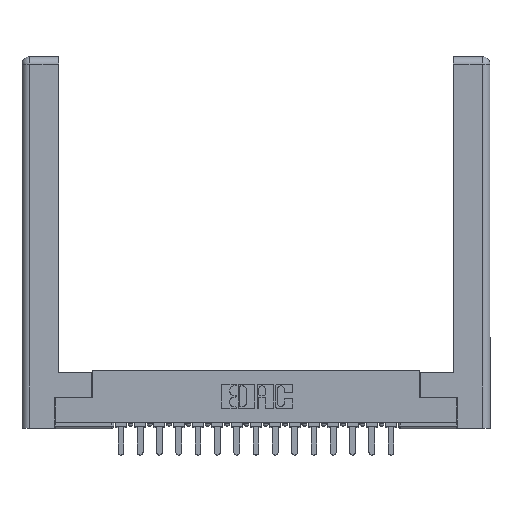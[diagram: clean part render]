
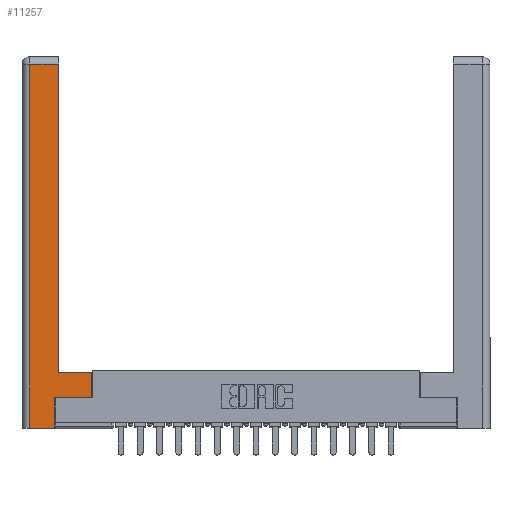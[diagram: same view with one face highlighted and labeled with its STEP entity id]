
A CAD part, top view. The second image highlights one B-rep face of the part: STEP entity #11257.
In plain terms, the highlighted planar face has unit normal (0, 0, 1).
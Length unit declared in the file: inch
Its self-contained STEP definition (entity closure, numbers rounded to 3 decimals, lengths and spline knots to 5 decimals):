
#6 = LINE ( 'NONE', #11619, #14843 ) ;
#325 = LINE ( 'NONE', #17585, #9475 ) ;
#982 = ORIENTED_EDGE ( 'NONE', *, *, #18937, .T. ) ;
#1104 = LINE ( 'NONE', #11465, #16669 ) ;
#1162 = LINE ( 'NONE', #10552, #17207 ) ;
#1489 = EDGE_LOOP ( 'NONE', ( #7624, #16201, #18060, #9174, #8798, #18848, #982, #4136 ) ) ;
#1714 = CARTESIAN_POINT ( 'NONE',  ( 0.295, 0.45, 0. ) ) ;
#1794 = EDGE_CURVE ( 'NONE', #12138, #5463, #15295, .T. ) ;
#2558 = CARTESIAN_POINT ( 'NONE',  ( 0.565, 0.45, 0. ) ) ;
#2696 = EDGE_CURVE ( 'NONE', #5463, #11904, #1104, .T. ) ;
#2821 = VERTEX_POINT ( 'NONE', #5671 ) ;
#2945 = CARTESIAN_POINT ( 'NONE',  ( 0.565, 0.45, 0. ) ) ;
#3159 = CARTESIAN_POINT ( 'NONE',  ( 0.565, 0.245, 0. ) ) ;
#3393 = DIRECTION ( 'NONE',  ( 0., -1., 0. ) ) ;
#3625 = EDGE_CURVE ( 'NONE', #17111, #4032, #6, .T. ) ;
#3726 = LINE ( 'NONE', #16613, #19297 ) ;
#3811 = DIRECTION ( 'NONE',  ( 0., 1., 0. ) ) ;
#3906 = VECTOR ( 'NONE', #3393, 39.37008 ) ;
#4023 = LINE ( 'NONE', #2945, #14396 ) ;
#4032 = VERTEX_POINT ( 'NONE', #18920 ) ;
#4136 = ORIENTED_EDGE ( 'NONE', *, *, #16254, .T. ) ;
#4484 = DIRECTION ( 'NONE',  ( 0., 1., 0. ) ) ;
#4532 = DIRECTION ( 'NONE',  ( 0., 1., 0. ) ) ;
#5429 = CARTESIAN_POINT ( 'NONE',  ( 0.265, 0., 0. ) ) ;
#5463 = VERTEX_POINT ( 'NONE', #11180 ) ;
#5554 = CARTESIAN_POINT ( 'NONE',  ( 0., 0., 0. ) ) ;
#5671 = CARTESIAN_POINT ( 'NONE',  ( 0.0615, 0., 0. ) ) ;
#6848 = AXIS2_PLACEMENT_3D ( 'NONE', #5554, #13160, #15858 ) ;
#7046 = EDGE_CURVE ( 'NONE', #7698, #17111, #1162, .T. ) ;
#7568 = DIRECTION ( 'NONE',  ( -1., 0., 0. ) ) ;
#7624 = ORIENTED_EDGE ( 'NONE', *, *, #7046, .T. ) ;
#7698 = VERTEX_POINT ( 'NONE', #1714 ) ;
#7746 = FACE_OUTER_BOUND ( 'NONE', #1489, .T. ) ;
#8323 = CARTESIAN_POINT ( 'NONE',  ( 0.265, 0.245, 0. ) ) ;
#8798 = ORIENTED_EDGE ( 'NONE', *, *, #1794, .T. ) ;
#9052 = CARTESIAN_POINT ( 'NONE',  ( 0.295, 2.94, 0. ) ) ;
#9174 = ORIENTED_EDGE ( 'NONE', *, *, #14680, .T. ) ;
#9475 = VECTOR ( 'NONE', #11384, 39.37008 ) ;
#9487 = EDGE_CURVE ( 'NONE', #4032, #2821, #11955, .T. ) ;
#10552 = CARTESIAN_POINT ( 'NONE',  ( 0.295, 3., 0. ) ) ;
#10849 = CARTESIAN_POINT ( 'NONE',  ( 0.0615, 0., 0. ) ) ;
#10889 = DIRECTION ( 'NONE',  ( -1., 0., 0. ) ) ;
#11180 = CARTESIAN_POINT ( 'NONE',  ( 0.265, 0.245, 0. ) ) ;
#11257 = ADVANCED_FACE ( 'NONE', ( #7746 ), #13026, .F. ) ;
#11384 = DIRECTION ( 'NONE',  ( 1., 0., 0. ) ) ;
#11465 = CARTESIAN_POINT ( 'NONE',  ( 0.565, 0.245, 0. ) ) ;
#11619 = CARTESIAN_POINT ( 'NONE',  ( 0.0615, 2.94, 0. ) ) ;
#11904 = VERTEX_POINT ( 'NONE', #3159 ) ;
#11955 = LINE ( 'NONE', #10849, #3906 ) ;
#12138 = VERTEX_POINT ( 'NONE', #5429 ) ;
#13026 = PLANE ( 'NONE',  #6848 ) ;
#13160 = DIRECTION ( 'NONE',  ( 0., 0., -1. ) ) ;
#14396 = VECTOR ( 'NONE', #4532, 39.37008 ) ;
#14680 = EDGE_CURVE ( 'NONE', #2821, #12138, #325, .T. ) ;
#14843 = VECTOR ( 'NONE', #7568, 39.37008 ) ;
#15295 = LINE ( 'NONE', #8323, #18578 ) ;
#15858 = DIRECTION ( 'NONE',  ( -1., 0., 0. ) ) ;
#16201 = ORIENTED_EDGE ( 'NONE', *, *, #3625, .T. ) ;
#16254 = EDGE_CURVE ( 'NONE', #18726, #7698, #3726, .T. ) ;
#16613 = CARTESIAN_POINT ( 'NONE',  ( 0.295, 0.45, 0. ) ) ;
#16669 = VECTOR ( 'NONE', #17397, 39.37008 ) ;
#17111 = VERTEX_POINT ( 'NONE', #9052 ) ;
#17207 = VECTOR ( 'NONE', #4484, 39.37008 ) ;
#17397 = DIRECTION ( 'NONE',  ( 1., 0., 0. ) ) ;
#17585 = CARTESIAN_POINT ( 'NONE',  ( 0.265, 0., 0. ) ) ;
#18060 = ORIENTED_EDGE ( 'NONE', *, *, #9487, .T. ) ;
#18578 = VECTOR ( 'NONE', #3811, 39.37008 ) ;
#18726 = VERTEX_POINT ( 'NONE', #2558 ) ;
#18848 = ORIENTED_EDGE ( 'NONE', *, *, #2696, .T. ) ;
#18920 = CARTESIAN_POINT ( 'NONE',  ( 0.0615, 2.94, 0. ) ) ;
#18937 = EDGE_CURVE ( 'NONE', #11904, #18726, #4023, .T. ) ;
#19297 = VECTOR ( 'NONE', #10889, 39.37008 ) ;
